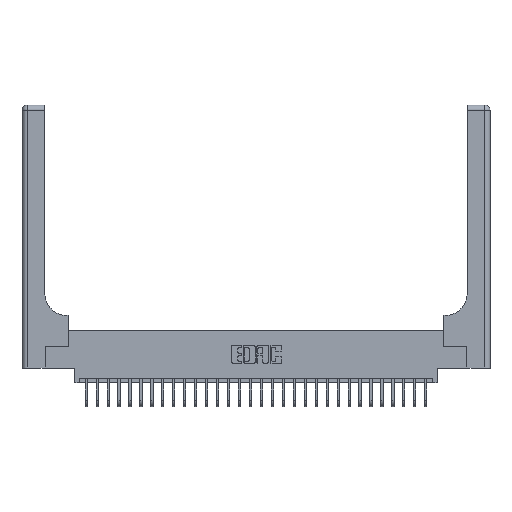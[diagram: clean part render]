
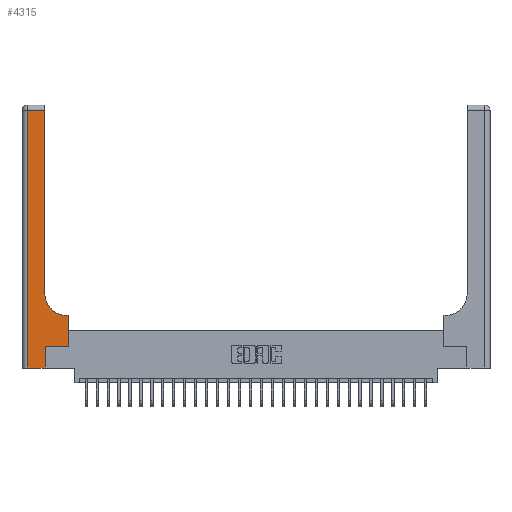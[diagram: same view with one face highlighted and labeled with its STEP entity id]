
A CAD part, top view. The second image highlights one B-rep face of the part: STEP entity #4315.
In plain terms, the highlighted planar face has unit normal (0, 0, 1).
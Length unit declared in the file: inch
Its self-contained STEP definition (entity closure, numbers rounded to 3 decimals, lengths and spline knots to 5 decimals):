
#170 = DIRECTION ( 'NONE',  ( 0., -1., 0. ) ) ;
#1054 = EDGE_LOOP ( 'NONE', ( #13752, #6091, #22803, #26727, #14630, #17559, #16928, #2934, #16745 ) ) ;
#1116 = CARTESIAN_POINT ( 'NONE',  ( 0.265, 0., 0.37 ) ) ;
#1126 = LINE ( 'NONE', #24452, #16549 ) ;
#1220 = VERTEX_POINT ( 'NONE', #22071 ) ;
#1542 = EDGE_CURVE ( 'NONE', #1220, #12814, #22950, .T. ) ;
#2401 = AXIS2_PLACEMENT_3D ( 'NONE', #7036, #4922, #2657 ) ;
#2582 = LINE ( 'NONE', #9359, #23001 ) ;
#2657 = DIRECTION ( 'NONE',  ( -1., 0., 0. ) ) ;
#2934 = ORIENTED_EDGE ( 'NONE', *, *, #24568, .T. ) ;
#3493 = CARTESIAN_POINT ( 'NONE',  ( 0.265, 0.25, 0.37 ) ) ;
#4315 = ADVANCED_FACE ( 'NONE', ( #12122 ), #20861, .F. ) ;
#4635 = DIRECTION ( 'NONE',  ( 1., 0., 0. ) ) ;
#4894 = VERTEX_POINT ( 'NONE', #28796 ) ;
#4922 = DIRECTION ( 'NONE',  ( 0., 0., -1. ) ) ;
#5238 = CARTESIAN_POINT ( 'NONE',  ( 0.26, 0.85, 0.37 ) ) ;
#5459 = DIRECTION ( 'NONE',  ( 1., 0., 0. ) ) ;
#6091 = ORIENTED_EDGE ( 'NONE', *, *, #7035, .T. ) ;
#6726 = CARTESIAN_POINT ( 'NONE',  ( 0.26, 3., 0.37 ) ) ;
#7026 = CARTESIAN_POINT ( 'NONE',  ( 0., 0., 0.37 ) ) ;
#7035 = EDGE_CURVE ( 'NONE', #20063, #21934, #1126, .T. ) ;
#7036 = CARTESIAN_POINT ( 'NONE',  ( 0., 3., 0.37 ) ) ;
#7262 = CARTESIAN_POINT ( 'NONE',  ( 0.51, 0.85, 0.37 ) ) ;
#8844 = DIRECTION ( 'NONE',  ( 0., 1., 0. ) ) ;
#9216 = DIRECTION ( 'NONE',  ( 0., 0., -1. ) ) ;
#9359 = CARTESIAN_POINT ( 'NONE',  ( 0.26, 0.6, 0.37 ) ) ;
#9587 = LINE ( 'NONE', #16073, #22084 ) ;
#9672 = EDGE_CURVE ( 'NONE', #15067, #20063, #10786, .T. ) ;
#10327 = DIRECTION ( 'NONE',  ( -1., 0., 0. ) ) ;
#10415 = CARTESIAN_POINT ( 'NONE',  ( 0.06, 2.94, 0.37 ) ) ;
#10785 = CARTESIAN_POINT ( 'NONE',  ( 0.528, 0.6, 0.37 ) ) ;
#10786 = LINE ( 'NONE', #6726, #11342 ) ;
#11342 = VECTOR ( 'NONE', #27193, 39.37008 ) ;
#12122 = FACE_OUTER_BOUND ( 'NONE', #1054, .T. ) ;
#12814 = VERTEX_POINT ( 'NONE', #1116 ) ;
#12859 = VECTOR ( 'NONE', #28653, 39.37008 ) ;
#13752 = ORIENTED_EDGE ( 'NONE', *, *, #9672, .T. ) ;
#14630 = ORIENTED_EDGE ( 'NONE', *, *, #21337, .T. ) ;
#15067 = VERTEX_POINT ( 'NONE', #5238 ) ;
#15501 = LINE ( 'NONE', #23954, #12859 ) ;
#16032 = AXIS2_PLACEMENT_3D ( 'NONE', #7262, #9216, #18255 ) ;
#16073 = CARTESIAN_POINT ( 'NONE',  ( 0.265, 0.25, 0.37 ) ) ;
#16443 = DIRECTION ( 'NONE',  ( -1., 0., 0. ) ) ;
#16549 = VECTOR ( 'NONE', #10327, 39.37008 ) ;
#16745 = ORIENTED_EDGE ( 'NONE', *, *, #22808, .T. ) ;
#16928 = ORIENTED_EDGE ( 'NONE', *, *, #20656, .T. ) ;
#17019 = CARTESIAN_POINT ( 'NONE',  ( 0.26, 2.94, 0.37 ) ) ;
#17559 = ORIENTED_EDGE ( 'NONE', *, *, #25361, .T. ) ;
#18255 = DIRECTION ( 'NONE',  ( 1., 0., 0. ) ) ;
#18628 = VECTOR ( 'NONE', #8844, 39.37008 ) ;
#20063 = VERTEX_POINT ( 'NONE', #17019 ) ;
#20254 = VERTEX_POINT ( 'NONE', #20905 ) ;
#20496 = CARTESIAN_POINT ( 'NONE',  ( 0.06, 3., 0.37 ) ) ;
#20569 = CARTESIAN_POINT ( 'NONE',  ( 0.528, 0.25, 0.37 ) ) ;
#20656 = EDGE_CURVE ( 'NONE', #4894, #22340, #20718, .T. ) ;
#20718 = LINE ( 'NONE', #20569, #18628 ) ;
#20861 = PLANE ( 'NONE',  #2401 ) ;
#20905 = CARTESIAN_POINT ( 'NONE',  ( 0.51, 0.6, 0.37 ) ) ;
#21337 = EDGE_CURVE ( 'NONE', #12814, #21905, #15501, .T. ) ;
#21777 = CIRCLE ( 'NONE', #16032, 0.25 ) ;
#21905 = VERTEX_POINT ( 'NONE', #3493 ) ;
#21934 = VERTEX_POINT ( 'NONE', #10415 ) ;
#22071 = CARTESIAN_POINT ( 'NONE',  ( 0.06, 0., 0.37 ) ) ;
#22084 = VECTOR ( 'NONE', #4635, 39.37008 ) ;
#22340 = VERTEX_POINT ( 'NONE', #10785 ) ;
#22803 = ORIENTED_EDGE ( 'NONE', *, *, #26330, .T. ) ;
#22808 = EDGE_CURVE ( 'NONE', #20254, #15067, #21777, .T. ) ;
#22950 = LINE ( 'NONE', #7026, #27172 ) ;
#23001 = VECTOR ( 'NONE', #16443, 39.37008 ) ;
#23954 = CARTESIAN_POINT ( 'NONE',  ( 0.265, 0., 0.37 ) ) ;
#24452 = CARTESIAN_POINT ( 'NONE',  ( 0., 2.94, 0.37 ) ) ;
#24568 = EDGE_CURVE ( 'NONE', #22340, #20254, #2582, .T. ) ;
#25361 = EDGE_CURVE ( 'NONE', #21905, #4894, #9587, .T. ) ;
#25463 = LINE ( 'NONE', #20496, #25977 ) ;
#25977 = VECTOR ( 'NONE', #170, 39.37008 ) ;
#26330 = EDGE_CURVE ( 'NONE', #21934, #1220, #25463, .T. ) ;
#26727 = ORIENTED_EDGE ( 'NONE', *, *, #1542, .T. ) ;
#27172 = VECTOR ( 'NONE', #5459, 39.37008 ) ;
#27193 = DIRECTION ( 'NONE',  ( 0., 1., 0. ) ) ;
#28653 = DIRECTION ( 'NONE',  ( 0., 1., 0. ) ) ;
#28796 = CARTESIAN_POINT ( 'NONE',  ( 0.528, 0.25, 0.37 ) ) ;
